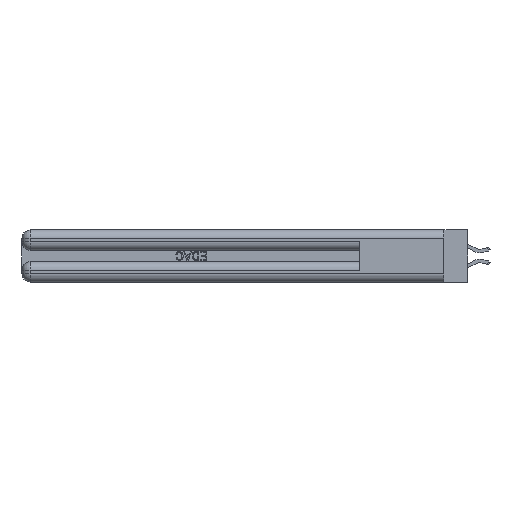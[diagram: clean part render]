
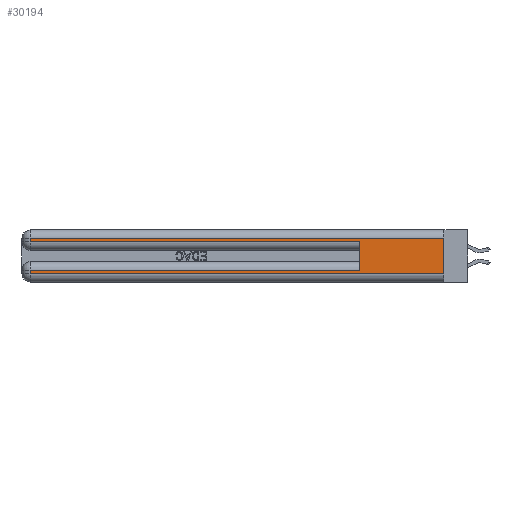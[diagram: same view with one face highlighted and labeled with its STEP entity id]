
A CAD part, left-side view. The second image highlights one B-rep face of the part: STEP entity #30194.
In plain terms, the highlighted planar face has unit normal (-1, 0, 0).
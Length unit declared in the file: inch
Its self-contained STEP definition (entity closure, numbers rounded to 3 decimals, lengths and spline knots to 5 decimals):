
#525 = LINE ( 'NONE', #23499, #13237 ) ;
#748 = VERTEX_POINT ( 'NONE', #7577 ) ;
#771 = VERTEX_POINT ( 'NONE', #7318 ) ;
#1444 = CARTESIAN_POINT ( 'NONE',  ( 0., 2.94, 0.085 ) ) ;
#3027 = AXIS2_PLACEMENT_3D ( 'NONE', #13725, #35287, #19938 ) ;
#4808 = ORIENTED_EDGE ( 'NONE', *, *, #18854, .T. ) ;
#4927 = VECTOR ( 'NONE', #35633, 39.37008 ) ;
#5376 = DIRECTION ( 'NONE',  ( 0., 1., 0. ) ) ;
#5727 = EDGE_CURVE ( 'NONE', #32075, #748, #15013, .T. ) ;
#6095 = ORIENTED_EDGE ( 'NONE', *, *, #20016, .T. ) ;
#6922 = CARTESIAN_POINT ( 'NONE',  ( 0., 0., 0.285 ) ) ;
#7318 = CARTESIAN_POINT ( 'NONE',  ( 0., 0., 0.06 ) ) ;
#7577 = CARTESIAN_POINT ( 'NONE',  ( 0., 2.94, 0.06 ) ) ;
#8311 = LINE ( 'NONE', #35059, #4927 ) ;
#9053 = CARTESIAN_POINT ( 'NONE',  ( 0., 2.94, 0.285 ) ) ;
#9354 = EDGE_CURVE ( 'NONE', #28515, #771, #16063, .T. ) ;
#10448 = EDGE_CURVE ( 'NONE', #30012, #30740, #38979, .T. ) ;
#10686 = VECTOR ( 'NONE', #12210, 39.37008 ) ;
#10767 = LINE ( 'NONE', #26863, #17655 ) ;
#11990 = CARTESIAN_POINT ( 'NONE',  ( 0., 2.94, 0.37 ) ) ;
#12210 = DIRECTION ( 'NONE',  ( 0., 0., -1. ) ) ;
#12232 = ORIENTED_EDGE ( 'NONE', *, *, #36431, .T. ) ;
#13237 = VECTOR ( 'NONE', #32862, 39.37008 ) ;
#13725 = CARTESIAN_POINT ( 'NONE',  ( 0., 0., 0.37 ) ) ;
#13967 = CARTESIAN_POINT ( 'NONE',  ( 0., 0.6, 0.145 ) ) ;
#14253 = DIRECTION ( 'NONE',  ( 0., 0., 1. ) ) ;
#14666 = VECTOR ( 'NONE', #18068, 39.37008 ) ;
#15013 = LINE ( 'NONE', #23190, #33570 ) ;
#15106 = EDGE_CURVE ( 'NONE', #28515, #27919, #8311, .T. ) ;
#16063 = LINE ( 'NONE', #34767, #10686 ) ;
#17655 = VECTOR ( 'NONE', #5376, 39.37008 ) ;
#18068 = DIRECTION ( 'NONE',  ( 0., 0., -1. ) ) ;
#18854 = EDGE_CURVE ( 'NONE', #748, #771, #525, .T. ) ;
#19165 = LINE ( 'NONE', #6922, #38193 ) ;
#19938 = DIRECTION ( 'NONE',  ( 0., 0., -1. ) ) ;
#20016 = EDGE_CURVE ( 'NONE', #27919, #22019, #26402, .T. ) ;
#20611 = CARTESIAN_POINT ( 'NONE',  ( 0., 0., 0.31 ) ) ;
#20694 = ORIENTED_EDGE ( 'NONE', *, *, #15106, .T. ) ;
#21092 = ORIENTED_EDGE ( 'NONE', *, *, #26194, .T. ) ;
#22019 = VERTEX_POINT ( 'NONE', #9053 ) ;
#22249 = CARTESIAN_POINT ( 'NONE',  ( 0., 0.6, 0.085 ) ) ;
#22333 = CARTESIAN_POINT ( 'NONE',  ( 0., 0.6, 0.285 ) ) ;
#23190 = CARTESIAN_POINT ( 'NONE',  ( 0., 2.94, 0.37 ) ) ;
#23499 = CARTESIAN_POINT ( 'NONE',  ( 0., 0., 0.06 ) ) ;
#23897 = DIRECTION ( 'NONE',  ( 0., 0., -1. ) ) ;
#24363 = VECTOR ( 'NONE', #14253, 39.37008 ) ;
#26194 = EDGE_CURVE ( 'NONE', #30012, #32075, #10767, .T. ) ;
#26402 = LINE ( 'NONE', #11990, #14666 ) ;
#26406 = FACE_OUTER_BOUND ( 'NONE', #39582, .T. ) ;
#26863 = CARTESIAN_POINT ( 'NONE',  ( 0., 0., 0.085 ) ) ;
#27919 = VERTEX_POINT ( 'NONE', #33277 ) ;
#28515 = VERTEX_POINT ( 'NONE', #20611 ) ;
#29035 = PLANE ( 'NONE',  #3027 ) ;
#30012 = VERTEX_POINT ( 'NONE', #22249 ) ;
#30194 = ADVANCED_FACE ( 'NONE', ( #26406 ), #29035, .F. ) ;
#30740 = VERTEX_POINT ( 'NONE', #22333 ) ;
#31537 = DIRECTION ( 'NONE',  ( 0., -1., 0. ) ) ;
#32075 = VERTEX_POINT ( 'NONE', #1444 ) ;
#32862 = DIRECTION ( 'NONE',  ( 0., -1., 0. ) ) ;
#33277 = CARTESIAN_POINT ( 'NONE',  ( 0., 2.94, 0.31 ) ) ;
#33339 = ORIENTED_EDGE ( 'NONE', *, *, #5727, .T. ) ;
#33570 = VECTOR ( 'NONE', #23897, 39.37008 ) ;
#34767 = CARTESIAN_POINT ( 'NONE',  ( 0., 0., 0.37 ) ) ;
#35059 = CARTESIAN_POINT ( 'NONE',  ( 0., 0., 0.31 ) ) ;
#35287 = DIRECTION ( 'NONE',  ( 1., 0., 0. ) ) ;
#35633 = DIRECTION ( 'NONE',  ( 0., 1., 0. ) ) ;
#36431 = EDGE_CURVE ( 'NONE', #22019, #30740, #19165, .T. ) ;
#37569 = ORIENTED_EDGE ( 'NONE', *, *, #10448, .F. ) ;
#38193 = VECTOR ( 'NONE', #31537, 39.37008 ) ;
#38979 = LINE ( 'NONE', #13967, #24363 ) ;
#39533 = ORIENTED_EDGE ( 'NONE', *, *, #9354, .F. ) ;
#39582 = EDGE_LOOP ( 'NONE', ( #39533, #20694, #6095, #12232, #37569, #21092, #33339, #4808 ) ) ;
